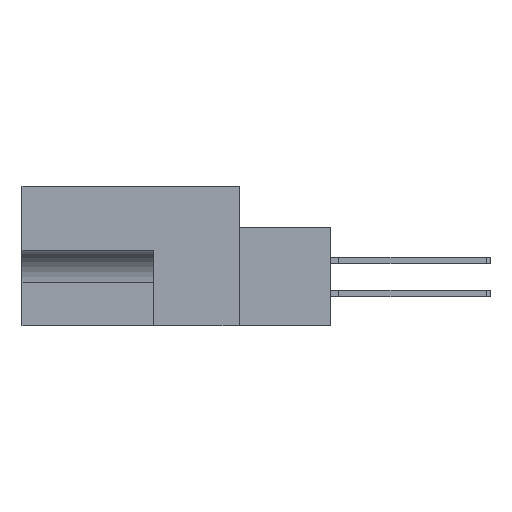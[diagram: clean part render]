
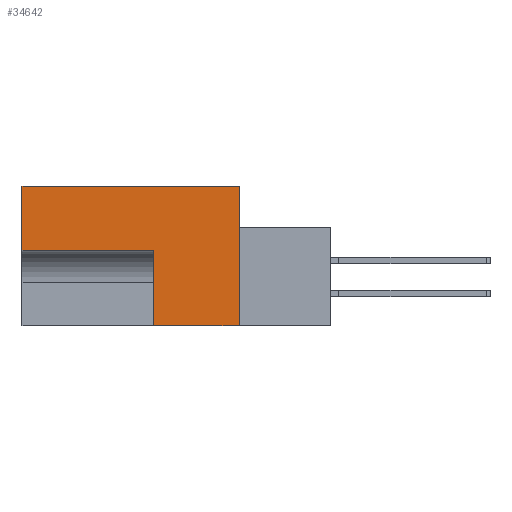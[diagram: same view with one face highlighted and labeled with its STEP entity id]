
A CAD part, left-side view. The second image highlights one B-rep face of the part: STEP entity #34642.
In plain terms, the highlighted planar face has unit normal (-1, 0, 0).
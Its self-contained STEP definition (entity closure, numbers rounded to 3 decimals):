
#155 = ORIENTED_EDGE ( 'NONE', *, *, #34034, .F. ) ;
#321 = VERTEX_POINT ( 'NONE', #39313 ) ;
#609 = EDGE_CURVE ( 'NONE', #14014, #21731, #2337, .T. ) ;
#839 = DIRECTION ( 'NONE',  ( 0., -1., 0. ) ) ;
#989 = DIRECTION ( 'NONE',  ( 0., 0., 1. ) ) ;
#1593 = LINE ( 'NONE', #34704, #2099 ) ;
#2079 = DIRECTION ( 'NONE',  ( 0., 1., 0. ) ) ;
#2099 = VECTOR ( 'NONE', #25215, 1000. ) ;
#2337 = LINE ( 'NONE', #19556, #18569 ) ;
#2526 = DIRECTION ( 'NONE',  ( 0., 1., 0. ) ) ;
#3558 = ORIENTED_EDGE ( 'NONE', *, *, #22268, .F. ) ;
#4022 = VECTOR ( 'NONE', #839, 1000. ) ;
#4236 = VECTOR ( 'NONE', #989, 1000. ) ;
#5029 = ORIENTED_EDGE ( 'NONE', *, *, #16814, .F. ) ;
#6794 = LINE ( 'NONE', #33497, #29984 ) ;
#9799 = CARTESIAN_POINT ( 'NONE',  ( 0., 20.955, 0. ) ) ;
#13237 = LINE ( 'NONE', #36088, #30028 ) ;
#14012 = CARTESIAN_POINT ( 'NONE',  ( 0., 0., 0. ) ) ;
#14014 = VERTEX_POINT ( 'NONE', #25459 ) ;
#16527 = LINE ( 'NONE', #19694, #4236 ) ;
#16814 = EDGE_CURVE ( 'NONE', #34550, #25160, #16527, .T. ) ;
#18569 = VECTOR ( 'NONE', #25382, 1000. ) ;
#19556 = CARTESIAN_POINT ( 'NONE',  ( 0., 0., 0. ) ) ;
#19694 = CARTESIAN_POINT ( 'NONE',  ( 0., 20.955, -13.487 ) ) ;
#20800 = CARTESIAN_POINT ( 'NONE',  ( 0., 0., -13.487 ) ) ;
#21731 = VERTEX_POINT ( 'NONE', #20800 ) ;
#22268 = EDGE_CURVE ( 'NONE', #321, #22474, #1593, .T. ) ;
#22474 = VERTEX_POINT ( 'NONE', #38128 ) ;
#23384 = PLANE ( 'NONE',  #37459 ) ;
#25155 = ORIENTED_EDGE ( 'NONE', *, *, #30411, .F. ) ;
#25160 = VERTEX_POINT ( 'NONE', #9799 ) ;
#25207 = LINE ( 'NONE', #38562, #4022 ) ;
#25215 = DIRECTION ( 'NONE',  ( 0., 0., 1. ) ) ;
#25285 = EDGE_CURVE ( 'NONE', #22474, #34550, #13237, .T. ) ;
#25382 = DIRECTION ( 'NONE',  ( 0., 0., -1. ) ) ;
#25459 = CARTESIAN_POINT ( 'NONE',  ( 0., 0., 0. ) ) ;
#25632 = FACE_OUTER_BOUND ( 'NONE', #32005, .T. ) ;
#29759 = DIRECTION ( 'NONE',  ( 0., 0., -1. ) ) ;
#29984 = VECTOR ( 'NONE', #2526, 1000. ) ;
#30028 = VECTOR ( 'NONE', #2079, 1000. ) ;
#30411 = EDGE_CURVE ( 'NONE', #21731, #321, #6794, .T. ) ;
#30417 = ORIENTED_EDGE ( 'NONE', *, *, #609, .F. ) ;
#32005 = EDGE_LOOP ( 'NONE', ( #25155, #30417, #155, #5029, #38321, #3558 ) ) ;
#32897 = DIRECTION ( 'NONE',  ( 1., 0., 0. ) ) ;
#33497 = CARTESIAN_POINT ( 'NONE',  ( 0., -8.814, -13.487 ) ) ;
#34034 = EDGE_CURVE ( 'NONE', #25160, #14014, #25207, .T. ) ;
#34550 = VERTEX_POINT ( 'NONE', #39351 ) ;
#34642 = ADVANCED_FACE ( 'NONE', ( #25632 ), #23384, .F. ) ;
#34704 = CARTESIAN_POINT ( 'NONE',  ( 0., 8.255, -13.487 ) ) ;
#36088 = CARTESIAN_POINT ( 'NONE',  ( 0., 8.255, -6.172 ) ) ;
#37459 = AXIS2_PLACEMENT_3D ( 'NONE', #14012, #32897, #29759 ) ;
#38128 = CARTESIAN_POINT ( 'NONE',  ( 0., 8.255, -6.172 ) ) ;
#38321 = ORIENTED_EDGE ( 'NONE', *, *, #25285, .F. ) ;
#38562 = CARTESIAN_POINT ( 'NONE',  ( 0., 11.506, 0. ) ) ;
#39313 = CARTESIAN_POINT ( 'NONE',  ( 0., 8.255, -13.487 ) ) ;
#39351 = CARTESIAN_POINT ( 'NONE',  ( 0., 20.955, -6.172 ) ) ;
